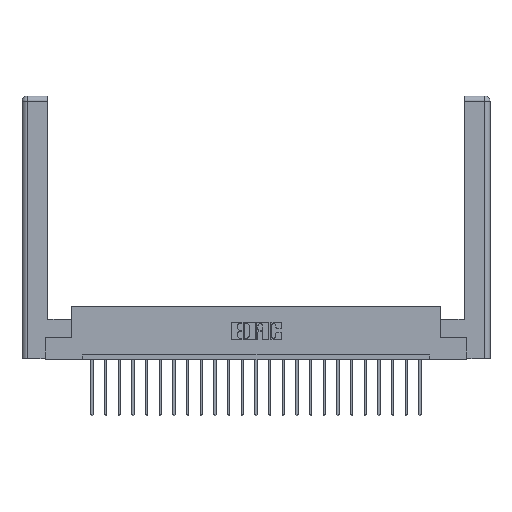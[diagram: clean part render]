
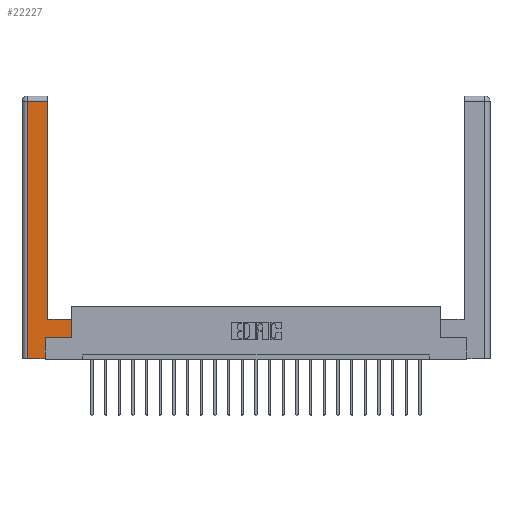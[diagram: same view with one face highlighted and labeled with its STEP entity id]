
A CAD part, top view. The second image highlights one B-rep face of the part: STEP entity #22227.
In plain terms, the highlighted planar face has unit normal (0, 0, 1).
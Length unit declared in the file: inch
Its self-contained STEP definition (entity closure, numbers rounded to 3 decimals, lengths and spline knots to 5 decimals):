
#27 = DIRECTION ( 'NONE',  ( -1., 0., 0. ) ) ;
#50 = LINE ( 'NONE', #14742, #16760 ) ;
#362 = VERTEX_POINT ( 'NONE', #15304 ) ;
#948 = CARTESIAN_POINT ( 'NONE',  ( 0.0615, 2.94, 0. ) ) ;
#1807 = CARTESIAN_POINT ( 'NONE',  ( 0.295, 2.94, 0. ) ) ;
#1813 = DIRECTION ( 'NONE',  ( 0., 1., 0. ) ) ;
#1819 = EDGE_CURVE ( 'NONE', #362, #22342, #17146, .T. ) ;
#2127 = CARTESIAN_POINT ( 'NONE',  ( 0.0615, 0., 0. ) ) ;
#2400 = LINE ( 'NONE', #948, #9502 ) ;
#2620 = DIRECTION ( 'NONE',  ( -1., 0., 0. ) ) ;
#2804 = VERTEX_POINT ( 'NONE', #13579 ) ;
#2849 = CARTESIAN_POINT ( 'NONE',  ( 0.0615, 0., 0. ) ) ;
#3214 = CARTESIAN_POINT ( 'NONE',  ( 0.265, 0.245, 0. ) ) ;
#3298 = CARTESIAN_POINT ( 'NONE',  ( 0.565, 0.245, 0. ) ) ;
#3739 = EDGE_LOOP ( 'NONE', ( #3920, #11303, #17702, #12370, #21661, #11427, #16054, #11676 ) ) ;
#3920 = ORIENTED_EDGE ( 'NONE', *, *, #1819, .T. ) ;
#4127 = LINE ( 'NONE', #18159, #14576 ) ;
#4895 = DIRECTION ( 'NONE',  ( 0., 0., -1. ) ) ;
#4982 = DIRECTION ( 'NONE',  ( 0., 1., 0. ) ) ;
#5047 = VERTEX_POINT ( 'NONE', #3214 ) ;
#5103 = CARTESIAN_POINT ( 'NONE',  ( 0.0615, 2.94, 0. ) ) ;
#5687 = VERTEX_POINT ( 'NONE', #5103 ) ;
#6295 = VERTEX_POINT ( 'NONE', #2127 ) ;
#6506 = VERTEX_POINT ( 'NONE', #19408 ) ;
#6784 = DIRECTION ( 'NONE',  ( 0., 1., 0. ) ) ;
#6965 = CARTESIAN_POINT ( 'NONE',  ( 0.565, 0.45, 0. ) ) ;
#7344 = EDGE_CURVE ( 'NONE', #6506, #12748, #4127, .T. ) ;
#9502 = VECTOR ( 'NONE', #2620, 39.37008 ) ;
#11079 = EDGE_CURVE ( 'NONE', #12748, #362, #50, .T. ) ;
#11303 = ORIENTED_EDGE ( 'NONE', *, *, #18945, .T. ) ;
#11427 = ORIENTED_EDGE ( 'NONE', *, *, #11697, .T. ) ;
#11676 = ORIENTED_EDGE ( 'NONE', *, *, #11079, .T. ) ;
#11697 = EDGE_CURVE ( 'NONE', #5047, #6506, #17008, .T. ) ;
#11921 = VECTOR ( 'NONE', #14600, 39.37008 ) ;
#12017 = LINE ( 'NONE', #16506, #17377 ) ;
#12177 = DIRECTION ( 'NONE',  ( -1., 0., 0. ) ) ;
#12370 = ORIENTED_EDGE ( 'NONE', *, *, #18258, .T. ) ;
#12728 = DIRECTION ( 'NONE',  ( 1., 0., 0. ) ) ;
#12748 = VERTEX_POINT ( 'NONE', #6965 ) ;
#13171 = LINE ( 'NONE', #2849, #23050 ) ;
#13579 = CARTESIAN_POINT ( 'NONE',  ( 0.265, 0., 0. ) ) ;
#13953 = CARTESIAN_POINT ( 'NONE',  ( 0.295, 3., 0. ) ) ;
#14021 = LINE ( 'NONE', #15634, #14306 ) ;
#14306 = VECTOR ( 'NONE', #4982, 39.37008 ) ;
#14576 = VECTOR ( 'NONE', #1813, 39.37008 ) ;
#14600 = DIRECTION ( 'NONE',  ( 1., 0., 0. ) ) ;
#14742 = CARTESIAN_POINT ( 'NONE',  ( 0.295, 0.45, 0. ) ) ;
#15304 = CARTESIAN_POINT ( 'NONE',  ( 0.295, 0.45, 0. ) ) ;
#15634 = CARTESIAN_POINT ( 'NONE',  ( 0.265, 0.245, 0. ) ) ;
#16054 = ORIENTED_EDGE ( 'NONE', *, *, #7344, .T. ) ;
#16506 = CARTESIAN_POINT ( 'NONE',  ( 0.265, 0., 0. ) ) ;
#16760 = VECTOR ( 'NONE', #27, 39.37008 ) ;
#17008 = LINE ( 'NONE', #3298, #11921 ) ;
#17146 = LINE ( 'NONE', #13953, #20274 ) ;
#17377 = VECTOR ( 'NONE', #12728, 39.37008 ) ;
#17693 = PLANE ( 'NONE',  #20555 ) ;
#17702 = ORIENTED_EDGE ( 'NONE', *, *, #18033, .T. ) ;
#18033 = EDGE_CURVE ( 'NONE', #5687, #6295, #13171, .T. ) ;
#18159 = CARTESIAN_POINT ( 'NONE',  ( 0.565, 0.45, 0. ) ) ;
#18258 = EDGE_CURVE ( 'NONE', #6295, #2804, #12017, .T. ) ;
#18544 = FACE_OUTER_BOUND ( 'NONE', #3739, .T. ) ;
#18945 = EDGE_CURVE ( 'NONE', #22342, #5687, #2400, .T. ) ;
#19408 = CARTESIAN_POINT ( 'NONE',  ( 0.565, 0.245, 0. ) ) ;
#20274 = VECTOR ( 'NONE', #6784, 39.37008 ) ;
#20555 = AXIS2_PLACEMENT_3D ( 'NONE', #21094, #4895, #12177 ) ;
#21094 = CARTESIAN_POINT ( 'NONE',  ( 0., 0., 0. ) ) ;
#21661 = ORIENTED_EDGE ( 'NONE', *, *, #22259, .T. ) ;
#22227 = ADVANCED_FACE ( 'NONE', ( #18544 ), #17693, .F. ) ;
#22259 = EDGE_CURVE ( 'NONE', #2804, #5047, #14021, .T. ) ;
#22342 = VERTEX_POINT ( 'NONE', #1807 ) ;
#23050 = VECTOR ( 'NONE', #23308, 39.37008 ) ;
#23308 = DIRECTION ( 'NONE',  ( 0., -1., 0. ) ) ;
